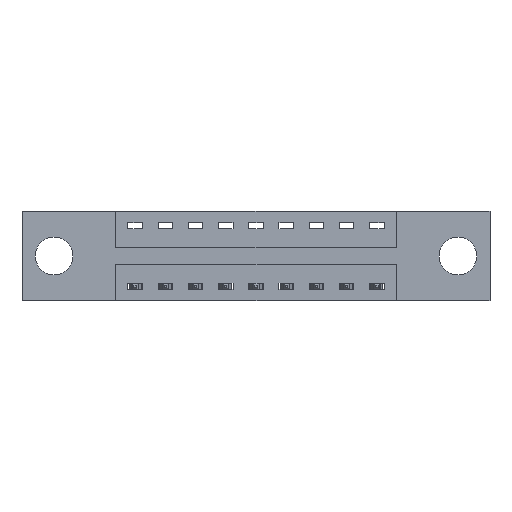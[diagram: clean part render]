
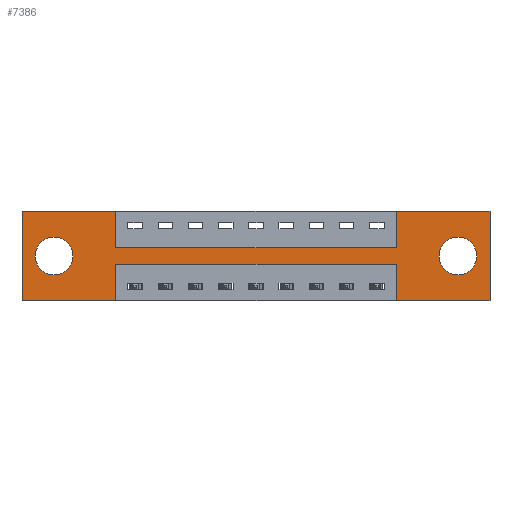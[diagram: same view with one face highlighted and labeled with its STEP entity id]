
A CAD part, front view. The second image highlights one B-rep face of the part: STEP entity #7386.
In plain terms, the highlighted planar face has unit normal (0, -1, 0).
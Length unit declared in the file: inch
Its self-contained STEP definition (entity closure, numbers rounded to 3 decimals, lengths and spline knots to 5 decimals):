
#26 = PLANE ( 'NONE',  #8797 ) ;
#102 = CIRCLE ( 'NONE', #6706, 0.078 ) ;
#181 = ORIENTED_EDGE ( 'NONE', *, *, #2221, .F. ) ;
#269 = LINE ( 'NONE', #7443, #6847 ) ;
#459 = DIRECTION ( 'NONE',  ( 0., 0., -1. ) ) ;
#475 = CARTESIAN_POINT ( 'NONE',  ( 1.5475, 0., -0.37 ) ) ;
#479 = LINE ( 'NONE', #2947, #4008 ) ;
#510 = AXIS2_PLACEMENT_3D ( 'NONE', #9148, #5074, #6128 ) ;
#536 = CARTESIAN_POINT ( 'NONE',  ( 0.3875, 0., -0.22 ) ) ;
#544 = ORIENTED_EDGE ( 'NONE', *, *, #7375, .T. ) ;
#606 = CARTESIAN_POINT ( 'NONE',  ( 1.935, 0., 0. ) ) ;
#694 = VECTOR ( 'NONE', #2665, 39.37008 ) ;
#807 = FACE_BOUND ( 'NONE', #9869, .T. ) ;
#1001 = DIRECTION ( 'NONE',  ( -1., 0., 0. ) ) ;
#1017 = VECTOR ( 'NONE', #2379, 39.37008 ) ;
#1057 = VERTEX_POINT ( 'NONE', #9154 ) ;
#1081 = EDGE_CURVE ( 'NONE', #8792, #2917, #269, .T. ) ;
#1105 = DIRECTION ( 'NONE',  ( 0., 0., -1. ) ) ;
#1202 = VECTOR ( 'NONE', #1001, 39.37008 ) ;
#1290 = CARTESIAN_POINT ( 'NONE',  ( 0., 0., 0. ) ) ;
#1451 = EDGE_CURVE ( 'NONE', #9893, #5618, #8952, .T. ) ;
#1523 = VECTOR ( 'NONE', #459, 39.37008 ) ;
#1570 = DIRECTION ( 'NONE',  ( 0., 0., -1. ) ) ;
#1665 = CARTESIAN_POINT ( 'NONE',  ( 1.935, 0., 0. ) ) ;
#1902 = CARTESIAN_POINT ( 'NONE',  ( 0., 0., -0.37 ) ) ;
#1918 = LINE ( 'NONE', #2916, #9122 ) ;
#1982 = LINE ( 'NONE', #606, #1523 ) ;
#2114 = CARTESIAN_POINT ( 'NONE',  ( 1.8025, 0., -0.107 ) ) ;
#2146 = EDGE_LOOP ( 'NONE', ( #8606, #5723, #5647, #8361, #3527, #4384, #4472, #3666, #5701, #6233, #7873, #181 ) ) ;
#2148 = CARTESIAN_POINT ( 'NONE',  ( 1.935, 0., -0.37 ) ) ;
#2213 = VERTEX_POINT ( 'NONE', #1665 ) ;
#2221 = EDGE_CURVE ( 'NONE', #6318, #2803, #9575, .T. ) ;
#2264 = CARTESIAN_POINT ( 'NONE',  ( 1.5475, 0., -0.37 ) ) ;
#2279 = DIRECTION ( 'NONE',  ( -1., 0., 0. ) ) ;
#2321 = DIRECTION ( 'NONE',  ( 0., 0., -1. ) ) ;
#2334 = EDGE_CURVE ( 'NONE', #1057, #9131, #102, .T. ) ;
#2379 = DIRECTION ( 'NONE',  ( 1., 0., 0. ) ) ;
#2558 = CARTESIAN_POINT ( 'NONE',  ( 1.5475, 0., 0. ) ) ;
#2665 = DIRECTION ( 'NONE',  ( 0., 0., 1. ) ) ;
#2667 = CIRCLE ( 'NONE', #2848, 0.078 ) ;
#2803 = VERTEX_POINT ( 'NONE', #6733 ) ;
#2818 = VECTOR ( 'NONE', #2279, 39.37008 ) ;
#2848 = AXIS2_PLACEMENT_3D ( 'NONE', #6473, #8835, #1570 ) ;
#2916 = CARTESIAN_POINT ( 'NONE',  ( 0., 0., 0. ) ) ;
#2917 = VERTEX_POINT ( 'NONE', #7665 ) ;
#2947 = CARTESIAN_POINT ( 'NONE',  ( 0.3875, 0., 0. ) ) ;
#2954 = DIRECTION ( 'NONE',  ( -1., 0., 0. ) ) ;
#3001 = AXIS2_PLACEMENT_3D ( 'NONE', #3627, #9229, #1105 ) ;
#3052 = DIRECTION ( 'NONE',  ( 0., 0., -1. ) ) ;
#3235 = CARTESIAN_POINT ( 'NONE',  ( 0., 0., -0.37 ) ) ;
#3270 = LINE ( 'NONE', #9763, #6029 ) ;
#3527 = ORIENTED_EDGE ( 'NONE', *, *, #9265, .F. ) ;
#3627 = CARTESIAN_POINT ( 'NONE',  ( 1.8025, 0., -0.185 ) ) ;
#3666 = ORIENTED_EDGE ( 'NONE', *, *, #1081, .F. ) ;
#3725 = CIRCLE ( 'NONE', #510, 0.078 ) ;
#3777 = VERTEX_POINT ( 'NONE', #8211 ) ;
#3932 = DIRECTION ( 'NONE',  ( 0., -1., 0. ) ) ;
#4008 = VECTOR ( 'NONE', #3052, 39.37008 ) ;
#4057 = FACE_BOUND ( 'NONE', #4490, .T. ) ;
#4384 = ORIENTED_EDGE ( 'NONE', *, *, #8157, .F. ) ;
#4396 = VERTEX_POINT ( 'NONE', #1290 ) ;
#4437 = VERTEX_POINT ( 'NONE', #8399 ) ;
#4472 = ORIENTED_EDGE ( 'NONE', *, *, #10440, .F. ) ;
#4490 = EDGE_LOOP ( 'NONE', ( #8908, #5476 ) ) ;
#4641 = DIRECTION ( 'NONE',  ( 0., 0., 1. ) ) ;
#4681 = EDGE_CURVE ( 'NONE', #4396, #3777, #3270, .T. ) ;
#4690 = LINE ( 'NONE', #475, #5244 ) ;
#4923 = EDGE_CURVE ( 'NONE', #3777, #8792, #479, .T. ) ;
#4952 = VERTEX_POINT ( 'NONE', #2148 ) ;
#5074 = DIRECTION ( 'NONE',  ( 0., 1., 0. ) ) ;
#5244 = VECTOR ( 'NONE', #4641, 39.37008 ) ;
#5476 = ORIENTED_EDGE ( 'NONE', *, *, #2334, .T. ) ;
#5595 = EDGE_CURVE ( 'NONE', #2803, #4396, #1918, .T. ) ;
#5618 = VERTEX_POINT ( 'NONE', #2114 ) ;
#5626 = EDGE_CURVE ( 'NONE', #7011, #6318, #6147, .T. ) ;
#5647 = ORIENTED_EDGE ( 'NONE', *, *, #10116, .F. ) ;
#5701 = ORIENTED_EDGE ( 'NONE', *, *, #4923, .F. ) ;
#5716 = CARTESIAN_POINT ( 'NONE',  ( 0., 0., 0. ) ) ;
#5723 = ORIENTED_EDGE ( 'NONE', *, *, #8376, .F. ) ;
#5826 = DIRECTION ( 'NONE',  ( 0., 0., 1. ) ) ;
#6029 = VECTOR ( 'NONE', #6562, 39.37008 ) ;
#6128 = DIRECTION ( 'NONE',  ( 0., 0., 1. ) ) ;
#6147 = LINE ( 'NONE', #8458, #8945 ) ;
#6233 = ORIENTED_EDGE ( 'NONE', *, *, #4681, .F. ) ;
#6303 = VERTEX_POINT ( 'NONE', #7323 ) ;
#6318 = VERTEX_POINT ( 'NONE', #9031 ) ;
#6407 = LINE ( 'NONE', #5716, #1017 ) ;
#6473 = CARTESIAN_POINT ( 'NONE',  ( 1.8025, 0., -0.185 ) ) ;
#6562 = DIRECTION ( 'NONE',  ( 1., 0., 0. ) ) ;
#6706 = AXIS2_PLACEMENT_3D ( 'NONE', #8929, #8349, #5826 ) ;
#6733 = CARTESIAN_POINT ( 'NONE',  ( 0., 0., -0.37 ) ) ;
#6809 = DIRECTION ( 'NONE',  ( 0., 0., -1. ) ) ;
#6847 = VECTOR ( 'NONE', #8239, 39.37008 ) ;
#7011 = VERTEX_POINT ( 'NONE', #8021 ) ;
#7299 = FACE_OUTER_BOUND ( 'NONE', #2146, .T. ) ;
#7323 = CARTESIAN_POINT ( 'NONE',  ( 1.5475, 0., -0.22 ) ) ;
#7375 = EDGE_CURVE ( 'NONE', #5618, #9893, #2667, .T. ) ;
#7386 = ADVANCED_FACE ( 'NONE', ( #807, #4057, #7299 ), #26, .T. ) ;
#7443 = CARTESIAN_POINT ( 'NONE',  ( 0.3875, 0., -0.15 ) ) ;
#7665 = CARTESIAN_POINT ( 'NONE',  ( 1.5475, 0., -0.15 ) ) ;
#7873 = ORIENTED_EDGE ( 'NONE', *, *, #5595, .F. ) ;
#8021 = CARTESIAN_POINT ( 'NONE',  ( 0.3875, 0., -0.22 ) ) ;
#8148 = CARTESIAN_POINT ( 'NONE',  ( 0., 0., -0.37 ) ) ;
#8157 = EDGE_CURVE ( 'NONE', #4437, #2213, #6407, .T. ) ;
#8211 = CARTESIAN_POINT ( 'NONE',  ( 0.3875, 0., 0. ) ) ;
#8239 = DIRECTION ( 'NONE',  ( 1., 0., 0. ) ) ;
#8349 = DIRECTION ( 'NONE',  ( 0., 1., 0. ) ) ;
#8361 = ORIENTED_EDGE ( 'NONE', *, *, #8696, .F. ) ;
#8376 = EDGE_CURVE ( 'NONE', #6303, #7011, #10286, .T. ) ;
#8399 = CARTESIAN_POINT ( 'NONE',  ( 1.5475, 0., 0. ) ) ;
#8458 = CARTESIAN_POINT ( 'NONE',  ( 0.3875, 0., -0.37 ) ) ;
#8479 = VERTEX_POINT ( 'NONE', #2264 ) ;
#8490 = CARTESIAN_POINT ( 'NONE',  ( 0.3875, 0., -0.15 ) ) ;
#8606 = ORIENTED_EDGE ( 'NONE', *, *, #5626, .F. ) ;
#8696 = EDGE_CURVE ( 'NONE', #4952, #8479, #9086, .T. ) ;
#8792 = VERTEX_POINT ( 'NONE', #8490 ) ;
#8797 = AXIS2_PLACEMENT_3D ( 'NONE', #3235, #3932, #2321 ) ;
#8815 = VECTOR ( 'NONE', #2954, 39.37008 ) ;
#8835 = DIRECTION ( 'NONE',  ( 0., 1., 0. ) ) ;
#8908 = ORIENTED_EDGE ( 'NONE', *, *, #10050, .T. ) ;
#8929 = CARTESIAN_POINT ( 'NONE',  ( 0.1325, 0., -0.185 ) ) ;
#8945 = VECTOR ( 'NONE', #6809, 39.37008 ) ;
#8952 = CIRCLE ( 'NONE', #3001, 0.078 ) ;
#9031 = CARTESIAN_POINT ( 'NONE',  ( 0.3875, 0., -0.37 ) ) ;
#9086 = LINE ( 'NONE', #1902, #1202 ) ;
#9122 = VECTOR ( 'NONE', #9418, 39.37008 ) ;
#9131 = VERTEX_POINT ( 'NONE', #9186 ) ;
#9148 = CARTESIAN_POINT ( 'NONE',  ( 0.1325, 0., -0.185 ) ) ;
#9154 = CARTESIAN_POINT ( 'NONE',  ( 0.1325, 0., -0.263 ) ) ;
#9186 = CARTESIAN_POINT ( 'NONE',  ( 0.1325, 0., -0.107 ) ) ;
#9229 = DIRECTION ( 'NONE',  ( 0., 1., 0. ) ) ;
#9265 = EDGE_CURVE ( 'NONE', #2213, #4952, #1982, .T. ) ;
#9418 = DIRECTION ( 'NONE',  ( 0., 0., 1. ) ) ;
#9575 = LINE ( 'NONE', #8148, #2818 ) ;
#9763 = CARTESIAN_POINT ( 'NONE',  ( 0., 0., 0. ) ) ;
#9869 = EDGE_LOOP ( 'NONE', ( #544, #10245 ) ) ;
#9893 = VERTEX_POINT ( 'NONE', #10065 ) ;
#10050 = EDGE_CURVE ( 'NONE', #9131, #1057, #3725, .T. ) ;
#10055 = LINE ( 'NONE', #2558, #694 ) ;
#10065 = CARTESIAN_POINT ( 'NONE',  ( 1.8025, 0., -0.263 ) ) ;
#10116 = EDGE_CURVE ( 'NONE', #8479, #6303, #4690, .T. ) ;
#10245 = ORIENTED_EDGE ( 'NONE', *, *, #1451, .T. ) ;
#10286 = LINE ( 'NONE', #536, #8815 ) ;
#10440 = EDGE_CURVE ( 'NONE', #2917, #4437, #10055, .T. ) ;
